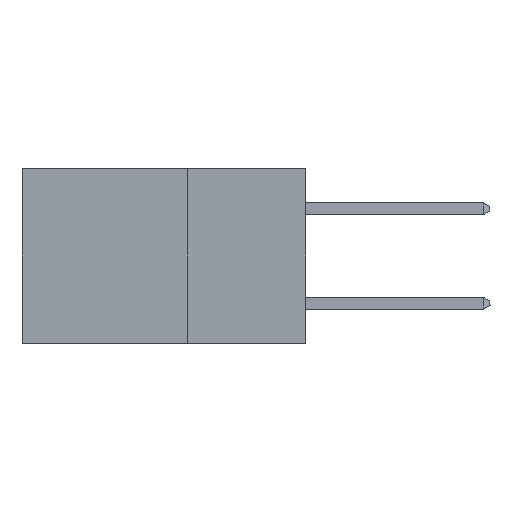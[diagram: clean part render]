
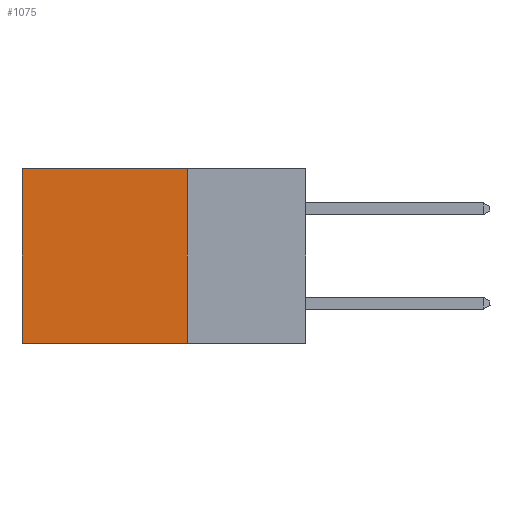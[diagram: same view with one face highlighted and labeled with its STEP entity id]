
A CAD part, left-side view. The second image highlights one B-rep face of the part: STEP entity #1075.
In plain terms, the highlighted planar face has unit normal (-1, 0, 0).
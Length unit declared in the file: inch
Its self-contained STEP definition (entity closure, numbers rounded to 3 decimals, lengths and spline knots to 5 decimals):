
#1075 = ADVANCED_FACE ( 'NONE', ( #23352 ), #22877, .F. ) ;
#1215 = CARTESIAN_POINT ( 'NONE',  ( 0.298, 0.25, 0. ) ) ;
#2768 = CARTESIAN_POINT ( 'NONE',  ( 0.298, 0.6, 0. ) ) ;
#3204 = VERTEX_POINT ( 'NONE', #25034 ) ;
#3377 = ORIENTED_EDGE ( 'NONE', *, *, #15877, .T. ) ;
#3518 = EDGE_CURVE ( 'NONE', #25175, #23671, #5498, .T. ) ;
#4090 = VECTOR ( 'NONE', #18394, 39.37008 ) ;
#4611 = ORIENTED_EDGE ( 'NONE', *, *, #22618, .F. ) ;
#5498 = LINE ( 'NONE', #13849, #22234 ) ;
#6850 = DIRECTION ( 'NONE',  ( 0., 1., 0. ) ) ;
#7632 = ORIENTED_EDGE ( 'NONE', *, *, #25719, .F. ) ;
#8068 = VECTOR ( 'NONE', #6850, 39.37008 ) ;
#8801 = ORIENTED_EDGE ( 'NONE', *, *, #3518, .T. ) ;
#9599 = DIRECTION ( 'NONE',  ( 0., 0., -1. ) ) ;
#10877 = VERTEX_POINT ( 'NONE', #17373 ) ;
#13849 = CARTESIAN_POINT ( 'NONE',  ( 0.298, 0.6, 0. ) ) ;
#13879 = DIRECTION ( 'NONE',  ( 0., 0., -1. ) ) ;
#14089 = VECTOR ( 'NONE', #25211, 39.37008 ) ;
#15877 = EDGE_CURVE ( 'NONE', #3204, #25175, #25543, .T. ) ;
#17373 = CARTESIAN_POINT ( 'NONE',  ( 0.298, 0.25, -0.37 ) ) ;
#18394 = DIRECTION ( 'NONE',  ( 0., 0., -1. ) ) ;
#19395 = AXIS2_PLACEMENT_3D ( 'NONE', #23015, #27695, #9599 ) ;
#19925 = CARTESIAN_POINT ( 'NONE',  ( 0.298, 0.25, -0.37 ) ) ;
#22234 = VECTOR ( 'NONE', #13879, 39.37008 ) ;
#22618 = EDGE_CURVE ( 'NONE', #3204, #10877, #26484, .T. ) ;
#22877 = PLANE ( 'NONE',  #19395 ) ;
#23015 = CARTESIAN_POINT ( 'NONE',  ( 0.298, 0.25, 0. ) ) ;
#23352 = FACE_OUTER_BOUND ( 'NONE', #26463, .T. ) ;
#23366 = LINE ( 'NONE', #19925, #8068 ) ;
#23671 = VERTEX_POINT ( 'NONE', #24375 ) ;
#24375 = CARTESIAN_POINT ( 'NONE',  ( 0.298, 0.6, -0.37 ) ) ;
#24867 = CARTESIAN_POINT ( 'NONE',  ( 0.298, 0.25, 0. ) ) ;
#25034 = CARTESIAN_POINT ( 'NONE',  ( 0.298, 0.25, 0. ) ) ;
#25175 = VERTEX_POINT ( 'NONE', #2768 ) ;
#25211 = DIRECTION ( 'NONE',  ( 0., 1., 0. ) ) ;
#25543 = LINE ( 'NONE', #1215, #14089 ) ;
#25719 = EDGE_CURVE ( 'NONE', #10877, #23671, #23366, .T. ) ;
#26463 = EDGE_LOOP ( 'NONE', ( #8801, #7632, #4611, #3377 ) ) ;
#26484 = LINE ( 'NONE', #24867, #4090 ) ;
#27695 = DIRECTION ( 'NONE',  ( 1., 0., 0. ) ) ;
